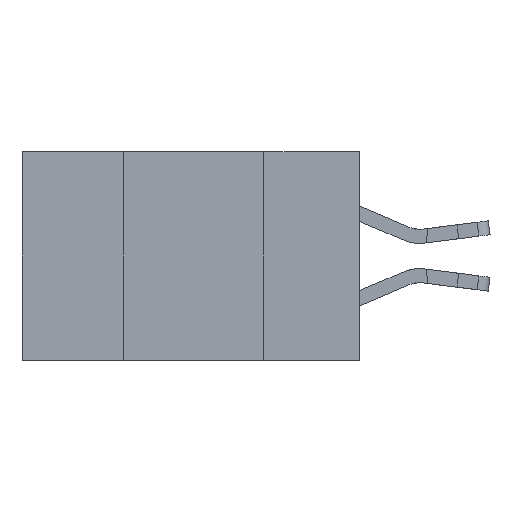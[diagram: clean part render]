
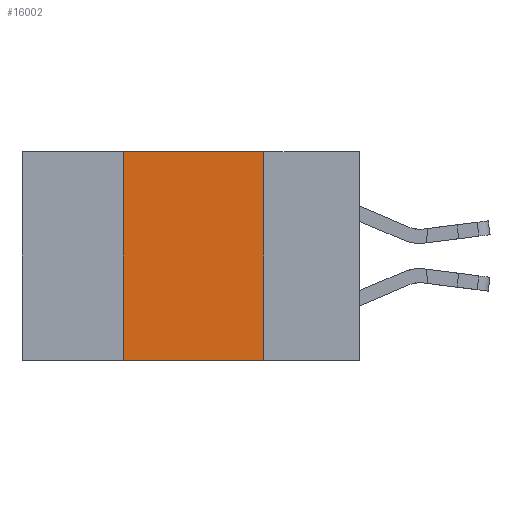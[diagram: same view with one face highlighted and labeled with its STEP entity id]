
A CAD part, left-side view. The second image highlights one B-rep face of the part: STEP entity #16002.
In plain terms, the highlighted planar face has unit normal (-1, 0, 0).
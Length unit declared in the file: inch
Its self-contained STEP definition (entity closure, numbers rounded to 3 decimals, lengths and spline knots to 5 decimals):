
#302 = VERTEX_POINT ( 'NONE', #794 ) ;
#466 = CARTESIAN_POINT ( 'NONE',  ( 0., 0.6, -0.37 ) ) ;
#794 = CARTESIAN_POINT ( 'NONE',  ( 0., 0.17, 0. ) ) ;
#1582 = VERTEX_POINT ( 'NONE', #3075 ) ;
#2178 = DIRECTION ( 'NONE',  ( 0., -1., 0. ) ) ;
#2481 = AXIS2_PLACEMENT_3D ( 'NONE', #8407, #20027, #10094 ) ;
#2830 = EDGE_LOOP ( 'NONE', ( #12004, #4465, #3556, #11140 ) ) ;
#3075 = CARTESIAN_POINT ( 'NONE',  ( 0., 0.42, -0.37 ) ) ;
#3095 = DIRECTION ( 'NONE',  ( 0., -1., 0. ) ) ;
#3254 = LINE ( 'NONE', #466, #16049 ) ;
#3556 = ORIENTED_EDGE ( 'NONE', *, *, #17485, .F. ) ;
#3943 = VECTOR ( 'NONE', #10442, 39.37008 ) ;
#4250 = LINE ( 'NONE', #14820, #8715 ) ;
#4465 = ORIENTED_EDGE ( 'NONE', *, *, #13985, .F. ) ;
#5005 = LINE ( 'NONE', #20340, #3943 ) ;
#5337 = CARTESIAN_POINT ( 'NONE',  ( 0., 0.17, 0. ) ) ;
#8220 = CARTESIAN_POINT ( 'NONE',  ( 0., 0.42, 0. ) ) ;
#8407 = CARTESIAN_POINT ( 'NONE',  ( 0., 0.6, 0. ) ) ;
#8715 = VECTOR ( 'NONE', #3095, 39.37008 ) ;
#10094 = DIRECTION ( 'NONE',  ( 0., 0., -1. ) ) ;
#10321 = DIRECTION ( 'NONE',  ( 0., 0., -1. ) ) ;
#10442 = DIRECTION ( 'NONE',  ( 0., 0., 1. ) ) ;
#11140 = ORIENTED_EDGE ( 'NONE', *, *, #20808, .T. ) ;
#12004 = ORIENTED_EDGE ( 'NONE', *, *, #14181, .F. ) ;
#13352 = VERTEX_POINT ( 'NONE', #8220 ) ;
#13446 = VECTOR ( 'NONE', #10321, 39.37008 ) ;
#13985 = EDGE_CURVE ( 'NONE', #13352, #302, #4250, .T. ) ;
#14181 = EDGE_CURVE ( 'NONE', #302, #21156, #17275, .T. ) ;
#14820 = CARTESIAN_POINT ( 'NONE',  ( 0., 0.6, 0. ) ) ;
#15631 = FACE_OUTER_BOUND ( 'NONE', #2830, .T. ) ;
#16002 = ADVANCED_FACE ( 'NONE', ( #15631 ), #16672, .F. ) ;
#16049 = VECTOR ( 'NONE', #2178, 39.37008 ) ;
#16672 = PLANE ( 'NONE',  #2481 ) ;
#17275 = LINE ( 'NONE', #5337, #13446 ) ;
#17485 = EDGE_CURVE ( 'NONE', #1582, #13352, #5005, .T. ) ;
#19877 = CARTESIAN_POINT ( 'NONE',  ( 0., 0.17, -0.37 ) ) ;
#20027 = DIRECTION ( 'NONE',  ( 1., 0., 0. ) ) ;
#20340 = CARTESIAN_POINT ( 'NONE',  ( 0., 0.42, 0. ) ) ;
#20808 = EDGE_CURVE ( 'NONE', #1582, #21156, #3254, .T. ) ;
#21156 = VERTEX_POINT ( 'NONE', #19877 ) ;
